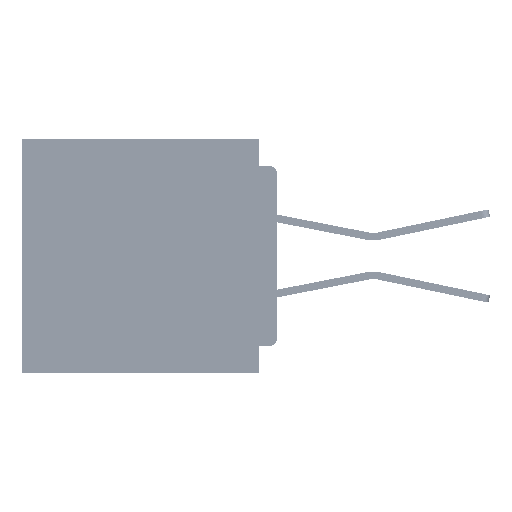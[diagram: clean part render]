
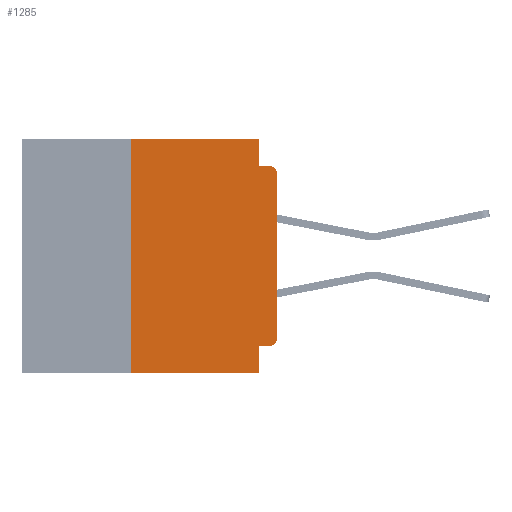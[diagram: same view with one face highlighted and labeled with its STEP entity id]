
A CAD part, left-side view. The second image highlights one B-rep face of the part: STEP entity #1285.
In plain terms, the highlighted planar face has unit normal (-1, 0, 0).
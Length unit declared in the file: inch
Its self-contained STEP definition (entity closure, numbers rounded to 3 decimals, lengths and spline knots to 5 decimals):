
#323 = AXIS2_PLACEMENT_3D ( 'NONE', #5336, #43482, #10874 ) ;
#738 = VERTEX_POINT ( 'NONE', #32987 ) ;
#1217 = CARTESIAN_POINT ( 'NONE',  ( 0., 0., -0.06 ) ) ;
#1285 = ADVANCED_FACE ( 'NONE', ( #40492 ), #53997, .F. ) ;
#1742 = EDGE_CURVE ( 'NONE', #58821, #41857, #11484, .T. ) ;
#2017 = ORIENTED_EDGE ( 'NONE', *, *, #22589, .F. ) ;
#2309 = DIRECTION ( 'NONE',  ( 0., -1., 0. ) ) ;
#2939 = VERTEX_POINT ( 'NONE', #2964 ) ;
#2964 = CARTESIAN_POINT ( 'NONE',  ( 0., 0.015, -0.355 ) ) ;
#3090 = VERTEX_POINT ( 'NONE', #47692 ) ;
#3830 = DIRECTION ( 'NONE',  ( 0., 0., 1. ) ) ;
#5336 = CARTESIAN_POINT ( 'NONE',  ( 0., 0.015, -0.06 ) ) ;
#5925 = VECTOR ( 'NONE', #61988, 39.37008 ) ;
#6397 = LINE ( 'NONE', #19399, #19241 ) ;
#6654 = EDGE_CURVE ( 'NONE', #40239, #50279, #69484, .T. ) ;
#7175 = CARTESIAN_POINT ( 'NONE',  ( 0., 0.031, -0.4 ) ) ;
#7783 = CARTESIAN_POINT ( 'NONE',  ( 0., 0.437, 0. ) ) ;
#9538 = ORIENTED_EDGE ( 'NONE', *, *, #53333, .F. ) ;
#10385 = CARTESIAN_POINT ( 'NONE',  ( 0., 0.031, 0. ) ) ;
#10715 = DIRECTION ( 'NONE',  ( 1., 0., 0. ) ) ;
#10874 = DIRECTION ( 'NONE',  ( 0., 0., -1. ) ) ;
#11484 = LINE ( 'NONE', #36517, #69260 ) ;
#12110 = VECTOR ( 'NONE', #40446, 39.37008 ) ;
#13446 = VECTOR ( 'NONE', #37548, 39.37008 ) ;
#14905 = EDGE_CURVE ( 'NONE', #67642, #40239, #26006, .T. ) ;
#14945 = CARTESIAN_POINT ( 'NONE',  ( 0., 0.031, -0.355 ) ) ;
#15545 = DIRECTION ( 'NONE',  ( 0., -1., 0. ) ) ;
#16326 = EDGE_CURVE ( 'NONE', #63055, #18458, #20680, .T. ) ;
#18458 = VERTEX_POINT ( 'NONE', #25028 ) ;
#19241 = VECTOR ( 'NONE', #30378, 39.37008 ) ;
#19399 = CARTESIAN_POINT ( 'NONE',  ( 0., 0.25, -0.4 ) ) ;
#20491 = LINE ( 'NONE', #29508, #5925 ) ;
#20680 = LINE ( 'NONE', #7175, #65703 ) ;
#22589 = EDGE_CURVE ( 'NONE', #50279, #3090, #55470, .T. ) ;
#22747 = ORIENTED_EDGE ( 'NONE', *, *, #51463, .T. ) ;
#24282 = VECTOR ( 'NONE', #2309, 39.37008 ) ;
#25028 = CARTESIAN_POINT ( 'NONE',  ( 0., 0.031, -0.4 ) ) ;
#26006 = LINE ( 'NONE', #7783, #24282 ) ;
#26509 = CARTESIAN_POINT ( 'NONE',  ( 0., 0.437, -0.4 ) ) ;
#29215 = AXIS2_PLACEMENT_3D ( 'NONE', #63298, #30840, #68738 ) ;
#29508 = CARTESIAN_POINT ( 'NONE',  ( 0., 0., -0.355 ) ) ;
#30378 = DIRECTION ( 'NONE',  ( 0., 0., 1. ) ) ;
#30811 = EDGE_CURVE ( 'NONE', #2939, #63055, #20491, .T. ) ;
#30840 = DIRECTION ( 'NONE',  ( -1., 0., 0. ) ) ;
#31478 = LINE ( 'NONE', #26509, #45882 ) ;
#32987 = CARTESIAN_POINT ( 'NONE',  ( 0., 0.25, -0.4 ) ) ;
#36517 = CARTESIAN_POINT ( 'NONE',  ( 0., 0., 0. ) ) ;
#37401 = CIRCLE ( 'NONE', #29215, 0.015 ) ;
#37548 = DIRECTION ( 'NONE',  ( 0., 0., -1. ) ) ;
#38911 = CIRCLE ( 'NONE', #323, 0.015 ) ;
#40239 = VERTEX_POINT ( 'NONE', #68245 ) ;
#40446 = DIRECTION ( 'NONE',  ( 0., -1., 0. ) ) ;
#40492 = FACE_OUTER_BOUND ( 'NONE', #53717, .T. ) ;
#41107 = EDGE_CURVE ( 'NONE', #41857, #3090, #38911, .T. ) ;
#41857 = VERTEX_POINT ( 'NONE', #1217 ) ;
#43482 = DIRECTION ( 'NONE',  ( -1., 0., 0. ) ) ;
#44267 = ORIENTED_EDGE ( 'NONE', *, *, #30811, .F. ) ;
#44934 = CARTESIAN_POINT ( 'NONE',  ( 0., 0.031, -0.045 ) ) ;
#45281 = DIRECTION ( 'NONE',  ( 0., 0., -1. ) ) ;
#45882 = VECTOR ( 'NONE', #15545, 39.37008 ) ;
#46526 = ORIENTED_EDGE ( 'NONE', *, *, #6654, .F. ) ;
#47692 = CARTESIAN_POINT ( 'NONE',  ( 0., 0.015, -0.045 ) ) ;
#48759 = DIRECTION ( 'NONE',  ( 0., 0., -1. ) ) ;
#50279 = VERTEX_POINT ( 'NONE', #44934 ) ;
#51463 = EDGE_CURVE ( 'NONE', #2939, #58821, #37401, .T. ) ;
#53167 = CARTESIAN_POINT ( 'NONE',  ( 0., 0.25, 0. ) ) ;
#53333 = EDGE_CURVE ( 'NONE', #738, #67642, #6397, .T. ) ;
#53587 = ORIENTED_EDGE ( 'NONE', *, *, #58496, .T. ) ;
#53717 = EDGE_LOOP ( 'NONE', ( #59134, #68069, #2017, #46526, #60234, #9538, #53587, #62790, #44267, #22747 ) ) ;
#53997 = PLANE ( 'NONE',  #62424 ) ;
#55470 = LINE ( 'NONE', #62279, #12110 ) ;
#55923 = CARTESIAN_POINT ( 'NONE',  ( 0., 0., -0.34 ) ) ;
#58496 = EDGE_CURVE ( 'NONE', #738, #18458, #31478, .T. ) ;
#58821 = VERTEX_POINT ( 'NONE', #55923 ) ;
#59134 = ORIENTED_EDGE ( 'NONE', *, *, #1742, .T. ) ;
#60234 = ORIENTED_EDGE ( 'NONE', *, *, #14905, .F. ) ;
#61988 = DIRECTION ( 'NONE',  ( 0., 1., 0. ) ) ;
#62279 = CARTESIAN_POINT ( 'NONE',  ( 0., 0., -0.045 ) ) ;
#62424 = AXIS2_PLACEMENT_3D ( 'NONE', #70306, #10715, #48759 ) ;
#62790 = ORIENTED_EDGE ( 'NONE', *, *, #16326, .F. ) ;
#63055 = VERTEX_POINT ( 'NONE', #14945 ) ;
#63298 = CARTESIAN_POINT ( 'NONE',  ( 0., 0.015, -0.34 ) ) ;
#65703 = VECTOR ( 'NONE', #45281, 39.37008 ) ;
#67642 = VERTEX_POINT ( 'NONE', #53167 ) ;
#68069 = ORIENTED_EDGE ( 'NONE', *, *, #41107, .T. ) ;
#68245 = CARTESIAN_POINT ( 'NONE',  ( 0., 0.031, 0. ) ) ;
#68738 = DIRECTION ( 'NONE',  ( 0., 0., -1. ) ) ;
#69260 = VECTOR ( 'NONE', #3830, 39.37008 ) ;
#69484 = LINE ( 'NONE', #10385, #13446 ) ;
#70306 = CARTESIAN_POINT ( 'NONE',  ( 0., 0.437, 0. ) ) ;
